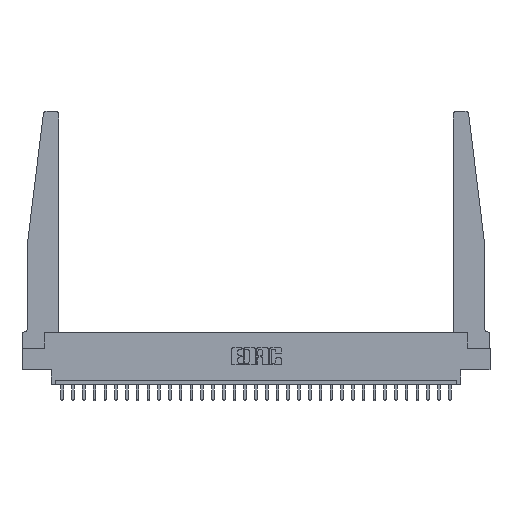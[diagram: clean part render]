
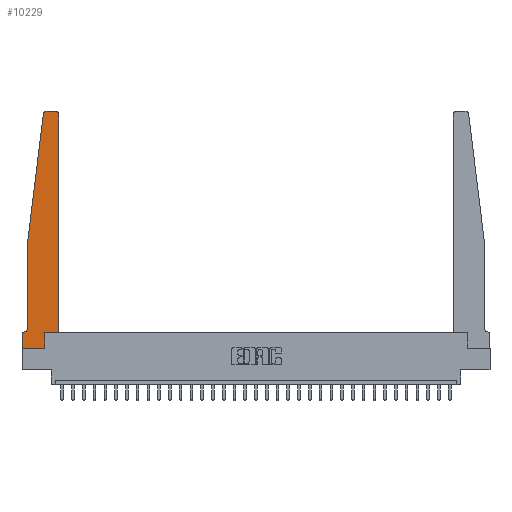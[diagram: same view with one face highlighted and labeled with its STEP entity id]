
A CAD part, top view. The second image highlights one B-rep face of the part: STEP entity #10229.
In plain terms, the highlighted planar face has unit normal (0, 0, 1).
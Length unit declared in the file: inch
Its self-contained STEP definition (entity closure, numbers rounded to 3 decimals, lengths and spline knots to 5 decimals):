
#475 = CIRCLE ( 'NONE', #23759, 0.03 ) ;
#529 = CARTESIAN_POINT ( 'NONE',  ( 0.27653, 2.72, 0.37 ) ) ;
#835 = EDGE_CURVE ( 'NONE', #1255, #3347, #23416, .T. ) ;
#982 = VECTOR ( 'NONE', #22735, 39.37008 ) ;
#1255 = VERTEX_POINT ( 'NONE', #11261 ) ;
#1426 = VERTEX_POINT ( 'NONE', #25449 ) ;
#1629 = CARTESIAN_POINT ( 'NONE',  ( 0.425, 0.18, 0.37 ) ) ;
#2097 = DIRECTION ( 'NONE',  ( 0., 1., 0. ) ) ;
#2564 = CARTESIAN_POINT ( 'NONE',  ( 0.395, 2.75, 0.37 ) ) ;
#2656 = VECTOR ( 'NONE', #2780, 39.37008 ) ;
#2780 = DIRECTION ( 'NONE',  ( 1., 0., 0. ) ) ;
#3347 = VERTEX_POINT ( 'NONE', #11150 ) ;
#3396 = VECTOR ( 'NONE', #15928, 39.37008 ) ;
#3740 = DIRECTION ( 'NONE',  ( 0., 0., 1. ) ) ;
#3944 = DIRECTION ( 'NONE',  ( -1., 0., 0. ) ) ;
#3994 = DIRECTION ( 'NONE',  ( 0., 0., 1. ) ) ;
#4280 = DIRECTION ( 'NONE',  ( 1., 0., 0. ) ) ;
#4640 = LINE ( 'NONE', #21544, #20886 ) ;
#4721 = CARTESIAN_POINT ( 'NONE',  ( 0., 0., 0.37 ) ) ;
#4787 = LINE ( 'NONE', #13962, #982 ) ;
#4930 = VERTEX_POINT ( 'NONE', #10623 ) ;
#5235 = EDGE_CURVE ( 'NONE', #4930, #22684, #20084, .T. ) ;
#5440 = LINE ( 'NONE', #1629, #20649 ) ;
#6105 = CARTESIAN_POINT ( 'NONE',  ( 0.425, 0.18, 0.37 ) ) ;
#6359 = ORIENTED_EDGE ( 'NONE', *, *, #27193, .T. ) ;
#6907 = AXIS2_PLACEMENT_3D ( 'NONE', #23763, #3740, #17024 ) ;
#7056 = VERTEX_POINT ( 'NONE', #16912 ) ;
#7286 = CARTESIAN_POINT ( 'NONE',  ( 0., 0.1875, 0.37 ) ) ;
#7856 = CIRCLE ( 'NONE', #6907, 0.03 ) ;
#8113 = VECTOR ( 'NONE', #10867, 39.37008 ) ;
#8452 = DIRECTION ( 'NONE',  ( 0., -1., 0. ) ) ;
#8470 = ORIENTED_EDGE ( 'NONE', *, *, #26329, .T. ) ;
#9103 = VECTOR ( 'NONE', #2097, 39.37008 ) ;
#9451 = DIRECTION ( 'NONE',  ( 0., 0., 1. ) ) ;
#9632 = CARTESIAN_POINT ( 'NONE',  ( 0.015, 0.1875, 0.37 ) ) ;
#9688 = CARTESIAN_POINT ( 'NONE',  ( 0.425, 0.18, 0.37 ) ) ;
#10203 = LINE ( 'NONE', #22163, #8113 ) ;
#10229 = ADVANCED_FACE ( 'NONE', ( #23145 ), #22994, .T. ) ;
#10623 = CARTESIAN_POINT ( 'NONE',  ( 0.065, 0.2375, 0.37 ) ) ;
#10814 = LINE ( 'NONE', #13316, #9103 ) ;
#10867 = DIRECTION ( 'NONE',  ( -0.122, -0.992, 0. ) ) ;
#11150 = CARTESIAN_POINT ( 'NONE',  ( 0.2605, 0., 0.37 ) ) ;
#11261 = CARTESIAN_POINT ( 'NONE',  ( 0., 0., 0.37 ) ) ;
#11995 = CARTESIAN_POINT ( 'NONE',  ( 0.065, 1.25, 0.37 ) ) ;
#12022 = CARTESIAN_POINT ( 'NONE',  ( 0., 0.1875, 0.37 ) ) ;
#12527 = ORIENTED_EDGE ( 'NONE', *, *, #17844, .T. ) ;
#12932 = VERTEX_POINT ( 'NONE', #2564 ) ;
#13316 = CARTESIAN_POINT ( 'NONE',  ( 0.2605, 0.18, 0.37 ) ) ;
#13646 = EDGE_CURVE ( 'NONE', #7056, #17486, #10203, .T. ) ;
#13791 = EDGE_CURVE ( 'NONE', #15930, #7056, #475, .T. ) ;
#13962 = CARTESIAN_POINT ( 'NONE',  ( 0.25, 2.75, 0.37 ) ) ;
#14009 = CARTESIAN_POINT ( 'NONE',  ( 0.065, 1.25, 0.37 ) ) ;
#14213 = ORIENTED_EDGE ( 'NONE', *, *, #27248, .T. ) ;
#14688 = DIRECTION ( 'NONE',  ( 0., 1., 0. ) ) ;
#14833 = LINE ( 'NONE', #11995, #18642 ) ;
#15122 = CARTESIAN_POINT ( 'NONE',  ( 0.2605, 0.18, 0.37 ) ) ;
#15308 = VERTEX_POINT ( 'NONE', #9688 ) ;
#15471 = DIRECTION ( 'NONE',  ( 0., 0., -1. ) ) ;
#15928 = DIRECTION ( 'NONE',  ( -1., 0., 0. ) ) ;
#15930 = VERTEX_POINT ( 'NONE', #27422 ) ;
#16789 = AXIS2_PLACEMENT_3D ( 'NONE', #26280, #15471, #3944 ) ;
#16877 = AXIS2_PLACEMENT_3D ( 'NONE', #12022, #3994, #4280 ) ;
#16912 = CARTESIAN_POINT ( 'NONE',  ( 0.24675, 2.72367, 0.37 ) ) ;
#17024 = DIRECTION ( 'NONE',  ( 1., 0., 0. ) ) ;
#17080 = ORIENTED_EDGE ( 'NONE', *, *, #21012, .T. ) ;
#17106 = ORIENTED_EDGE ( 'NONE', *, *, #27162, .T. ) ;
#17486 = VERTEX_POINT ( 'NONE', #14009 ) ;
#17608 = ORIENTED_EDGE ( 'NONE', *, *, #20969, .T. ) ;
#17844 = EDGE_CURVE ( 'NONE', #27969, #1255, #4640, .T. ) ;
#18262 = LINE ( 'NONE', #6105, #21314 ) ;
#18503 = DIRECTION ( 'NONE',  ( 0., -1., 0. ) ) ;
#18642 = VECTOR ( 'NONE', #18503, 39.37008 ) ;
#20084 = CIRCLE ( 'NONE', #16789, 0.05 ) ;
#20250 = VERTEX_POINT ( 'NONE', #15122 ) ;
#20649 = VECTOR ( 'NONE', #14688, 39.37008 ) ;
#20886 = VECTOR ( 'NONE', #8452, 39.37008 ) ;
#20969 = EDGE_CURVE ( 'NONE', #17486, #4930, #14833, .T. ) ;
#21012 = EDGE_CURVE ( 'NONE', #12932, #15930, #4787, .T. ) ;
#21314 = VECTOR ( 'NONE', #23860, 39.37008 ) ;
#21512 = ORIENTED_EDGE ( 'NONE', *, *, #835, .T. ) ;
#21544 = CARTESIAN_POINT ( 'NONE',  ( 0., 0., 0.37 ) ) ;
#22146 = EDGE_LOOP ( 'NONE', ( #17080, #25773, #28320, #17608, #23052, #8470, #12527, #21512, #27684, #17106, #6359, #14213 ) ) ;
#22163 = CARTESIAN_POINT ( 'NONE',  ( 0.065, 1.25, 0.37 ) ) ;
#22684 = VERTEX_POINT ( 'NONE', #9632 ) ;
#22735 = DIRECTION ( 'NONE',  ( -1., 0., 0. ) ) ;
#22994 = PLANE ( 'NONE',  #16877 ) ;
#23052 = ORIENTED_EDGE ( 'NONE', *, *, #5235, .T. ) ;
#23145 = FACE_OUTER_BOUND ( 'NONE', #22146, .T. ) ;
#23416 = LINE ( 'NONE', #4721, #2656 ) ;
#23759 = AXIS2_PLACEMENT_3D ( 'NONE', #529, #9451, #24618 ) ;
#23763 = CARTESIAN_POINT ( 'NONE',  ( 0.395, 2.72, 0.37 ) ) ;
#23837 = EDGE_CURVE ( 'NONE', #3347, #20250, #10814, .T. ) ;
#23860 = DIRECTION ( 'NONE',  ( 1., 0., 0. ) ) ;
#24166 = LINE ( 'NONE', #24805, #3396 ) ;
#24618 = DIRECTION ( 'NONE',  ( 1., 0., 0. ) ) ;
#24805 = CARTESIAN_POINT ( 'NONE',  ( 0.065, 0.1875, 0.37 ) ) ;
#25449 = CARTESIAN_POINT ( 'NONE',  ( 0.425, 2.72, 0.37 ) ) ;
#25773 = ORIENTED_EDGE ( 'NONE', *, *, #13791, .T. ) ;
#26280 = CARTESIAN_POINT ( 'NONE',  ( 0.015, 0.2375, 0.37 ) ) ;
#26329 = EDGE_CURVE ( 'NONE', #22684, #27969, #24166, .T. ) ;
#27162 = EDGE_CURVE ( 'NONE', #20250, #15308, #18262, .T. ) ;
#27193 = EDGE_CURVE ( 'NONE', #15308, #1426, #5440, .T. ) ;
#27248 = EDGE_CURVE ( 'NONE', #1426, #12932, #7856, .T. ) ;
#27422 = CARTESIAN_POINT ( 'NONE',  ( 0.27653, 2.75, 0.37 ) ) ;
#27684 = ORIENTED_EDGE ( 'NONE', *, *, #23837, .T. ) ;
#27969 = VERTEX_POINT ( 'NONE', #7286 ) ;
#28320 = ORIENTED_EDGE ( 'NONE', *, *, #13646, .T. ) ;
